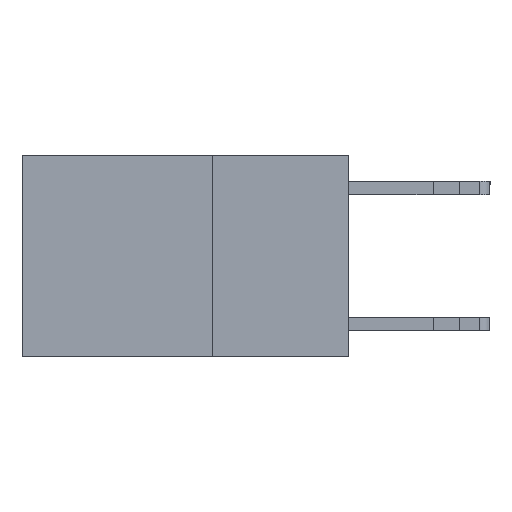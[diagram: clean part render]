
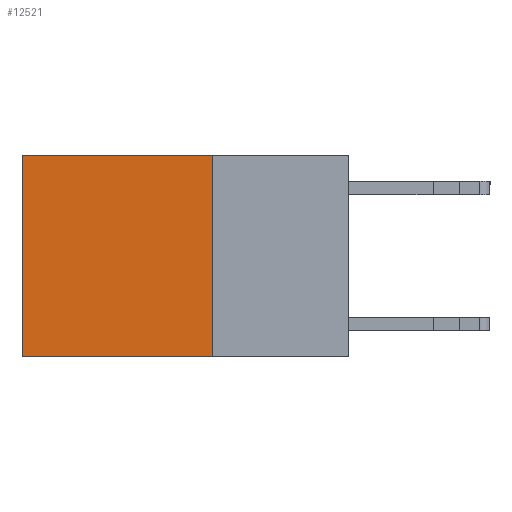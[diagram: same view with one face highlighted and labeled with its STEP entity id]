
A CAD part, left-side view. The second image highlights one B-rep face of the part: STEP entity #12521.
In plain terms, the highlighted planar face has unit normal (-1, 0, 0).
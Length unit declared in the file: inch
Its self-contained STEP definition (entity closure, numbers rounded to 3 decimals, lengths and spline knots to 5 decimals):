
#991 = CARTESIAN_POINT ( 'NONE',  ( 0.2625, 0.6, 0. ) ) ;
#1755 = VECTOR ( 'NONE', #2174, 39.37008 ) ;
#1925 = EDGE_LOOP ( 'NONE', ( #11560, #10828, #8848, #8362 ) ) ;
#2174 = DIRECTION ( 'NONE',  ( 0., 1., 0. ) ) ;
#2356 = DIRECTION ( 'NONE',  ( 0., 0., -1. ) ) ;
#2494 = VECTOR ( 'NONE', #12633, 39.37008 ) ;
#2645 = CARTESIAN_POINT ( 'NONE',  ( 0.2625, 0.25, 0. ) ) ;
#3247 = EDGE_CURVE ( 'NONE', #13707, #7215, #3532, .T. ) ;
#3532 = LINE ( 'NONE', #12541, #1755 ) ;
#3723 = EDGE_CURVE ( 'NONE', #7215, #4555, #4716, .T. ) ;
#3799 = DIRECTION ( 'NONE',  ( 0., 0., -1. ) ) ;
#4555 = VERTEX_POINT ( 'NONE', #6486 ) ;
#4628 = EDGE_CURVE ( 'NONE', #9567, #4555, #9982, .T. ) ;
#4716 = LINE ( 'NONE', #12748, #11398 ) ;
#5969 = PLANE ( 'NONE',  #7886 ) ;
#6486 = CARTESIAN_POINT ( 'NONE',  ( 0.2625, 0.6, -0.37 ) ) ;
#6563 = CARTESIAN_POINT ( 'NONE',  ( 0.2625, 0.25, -0.37 ) ) ;
#6951 = LINE ( 'NONE', #10715, #9358 ) ;
#7215 = VERTEX_POINT ( 'NONE', #991 ) ;
#7311 = EDGE_CURVE ( 'NONE', #13707, #9567, #6951, .T. ) ;
#7886 = AXIS2_PLACEMENT_3D ( 'NONE', #2645, #10588, #14219 ) ;
#8251 = FACE_OUTER_BOUND ( 'NONE', #1925, .T. ) ;
#8280 = CARTESIAN_POINT ( 'NONE',  ( 0.2625, 0.25, -0.37 ) ) ;
#8362 = ORIENTED_EDGE ( 'NONE', *, *, #3247, .T. ) ;
#8848 = ORIENTED_EDGE ( 'NONE', *, *, #7311, .F. ) ;
#8958 = CARTESIAN_POINT ( 'NONE',  ( 0.2625, 0.25, 0. ) ) ;
#9358 = VECTOR ( 'NONE', #2356, 39.37008 ) ;
#9567 = VERTEX_POINT ( 'NONE', #8280 ) ;
#9982 = LINE ( 'NONE', #6563, #2494 ) ;
#10588 = DIRECTION ( 'NONE',  ( 1., 0., 0. ) ) ;
#10715 = CARTESIAN_POINT ( 'NONE',  ( 0.2625, 0.25, 0. ) ) ;
#10828 = ORIENTED_EDGE ( 'NONE', *, *, #4628, .F. ) ;
#11398 = VECTOR ( 'NONE', #3799, 39.37008 ) ;
#11560 = ORIENTED_EDGE ( 'NONE', *, *, #3723, .T. ) ;
#12521 = ADVANCED_FACE ( 'NONE', ( #8251 ), #5969, .F. ) ;
#12541 = CARTESIAN_POINT ( 'NONE',  ( 0.2625, 0.25, 0. ) ) ;
#12633 = DIRECTION ( 'NONE',  ( 0., 1., 0. ) ) ;
#12748 = CARTESIAN_POINT ( 'NONE',  ( 0.2625, 0.6, 0. ) ) ;
#13707 = VERTEX_POINT ( 'NONE', #8958 ) ;
#14219 = DIRECTION ( 'NONE',  ( 0., 0., -1. ) ) ;
